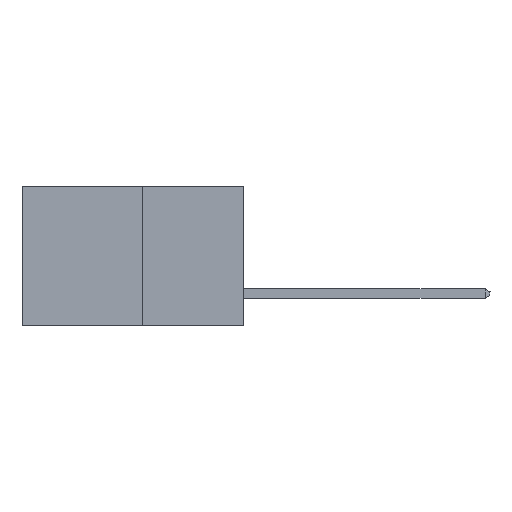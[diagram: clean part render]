
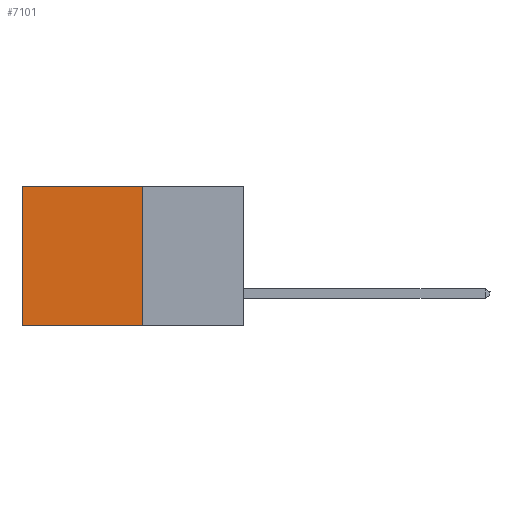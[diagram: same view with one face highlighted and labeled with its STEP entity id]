
A CAD part, left-side view. The second image highlights one B-rep face of the part: STEP entity #7101.
In plain terms, the highlighted planar face has unit normal (-1, 0, 0).
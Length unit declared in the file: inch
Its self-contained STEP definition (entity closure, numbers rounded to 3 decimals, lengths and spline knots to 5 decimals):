
#105 = EDGE_LOOP ( 'NONE', ( #15849, #705, #7300, #10593 ) ) ;
#172 = EDGE_CURVE ( 'NONE', #13575, #14759, #2658, .T. ) ;
#705 = ORIENTED_EDGE ( 'NONE', *, *, #172, .F. ) ;
#914 = VERTEX_POINT ( 'NONE', #3999 ) ;
#1341 = EDGE_CURVE ( 'NONE', #14567, #14759, #8021, .T. ) ;
#1836 = EDGE_CURVE ( 'NONE', #914, #14567, #3017, .T. ) ;
#2658 = LINE ( 'NONE', #11697, #5887 ) ;
#3017 = LINE ( 'NONE', #12525, #14608 ) ;
#3999 = CARTESIAN_POINT ( 'NONE',  ( 0.277, 0.27, 0. ) ) ;
#4548 = DIRECTION ( 'NONE',  ( 0., 0., -1. ) ) ;
#5887 = VECTOR ( 'NONE', #12928, 39.37008 ) ;
#6155 = DIRECTION ( 'NONE',  ( 0., 0., -1. ) ) ;
#7101 = ADVANCED_FACE ( 'NONE', ( #14073 ), #15581, .F. ) ;
#7300 = ORIENTED_EDGE ( 'NONE', *, *, #8017, .F. ) ;
#7644 = CARTESIAN_POINT ( 'NONE',  ( 0.277, 0.27, -0.37 ) ) ;
#7992 = CARTESIAN_POINT ( 'NONE',  ( 0.277, 0.59, 0. ) ) ;
#8017 = EDGE_CURVE ( 'NONE', #914, #13575, #9392, .T. ) ;
#8021 = LINE ( 'NONE', #11776, #15045 ) ;
#8356 = CARTESIAN_POINT ( 'NONE',  ( 0.277, 0.59, -0.37 ) ) ;
#8963 = VECTOR ( 'NONE', #6155, 39.37008 ) ;
#9392 = LINE ( 'NONE', #7644, #8963 ) ;
#10593 = ORIENTED_EDGE ( 'NONE', *, *, #1836, .T. ) ;
#11322 = DIRECTION ( 'NONE',  ( 0., 1., 0. ) ) ;
#11697 = CARTESIAN_POINT ( 'NONE',  ( 0.277, 0.27, -0.37 ) ) ;
#11776 = CARTESIAN_POINT ( 'NONE',  ( 0.277, 0.59, -0.37 ) ) ;
#12010 = AXIS2_PLACEMENT_3D ( 'NONE', #14737, #14727, #14707 ) ;
#12525 = CARTESIAN_POINT ( 'NONE',  ( 0.277, 0.27, 0. ) ) ;
#12928 = DIRECTION ( 'NONE',  ( 0., 1., 0. ) ) ;
#13575 = VERTEX_POINT ( 'NONE', #16256 ) ;
#14073 = FACE_OUTER_BOUND ( 'NONE', #105, .T. ) ;
#14567 = VERTEX_POINT ( 'NONE', #7992 ) ;
#14608 = VECTOR ( 'NONE', #11322, 39.37008 ) ;
#14707 = DIRECTION ( 'NONE',  ( 0., 0., -1. ) ) ;
#14727 = DIRECTION ( 'NONE',  ( 1., 0., 0. ) ) ;
#14737 = CARTESIAN_POINT ( 'NONE',  ( 0.277, 0.27, -0.37 ) ) ;
#14759 = VERTEX_POINT ( 'NONE', #8356 ) ;
#15045 = VECTOR ( 'NONE', #4548, 39.37008 ) ;
#15581 = PLANE ( 'NONE',  #12010 ) ;
#15849 = ORIENTED_EDGE ( 'NONE', *, *, #1341, .T. ) ;
#16256 = CARTESIAN_POINT ( 'NONE',  ( 0.277, 0.27, -0.37 ) ) ;
